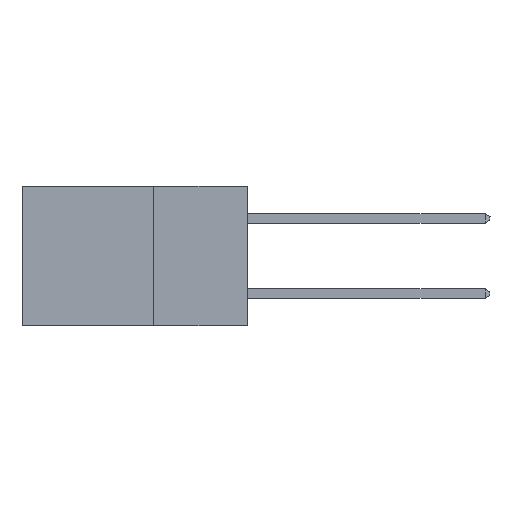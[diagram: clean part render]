
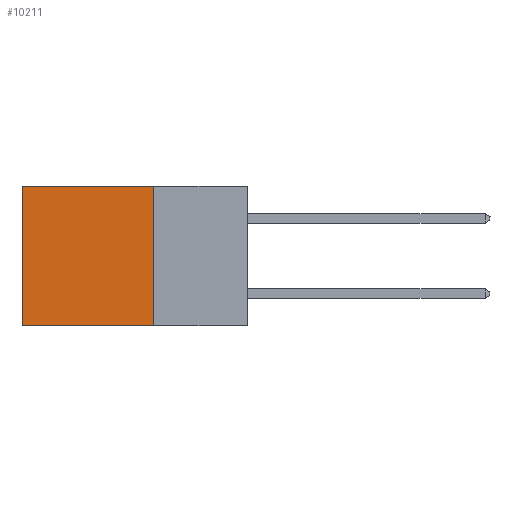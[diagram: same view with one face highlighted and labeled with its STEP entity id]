
A CAD part, left-side view. The second image highlights one B-rep face of the part: STEP entity #10211.
In plain terms, the highlighted planar face has unit normal (-1, 0, 0).
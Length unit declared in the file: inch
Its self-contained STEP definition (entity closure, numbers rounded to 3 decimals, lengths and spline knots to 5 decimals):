
#369 = CARTESIAN_POINT ( 'NONE',  ( 0.298, 0.25, 0. ) ) ;
#521 = LINE ( 'NONE', #3110, #3900 ) ;
#1960 = ORIENTED_EDGE ( 'NONE', *, *, #22011, .T. ) ;
#2977 = DIRECTION ( 'NONE',  ( 0., 0., -1. ) ) ;
#3110 = CARTESIAN_POINT ( 'NONE',  ( 0.298, 0.6, 0. ) ) ;
#3223 = EDGE_CURVE ( 'NONE', #9726, #11588, #18901, .T. ) ;
#3747 = CARTESIAN_POINT ( 'NONE',  ( 0.298, 0.25, -0.37 ) ) ;
#3900 = VECTOR ( 'NONE', #24812, 39.37008 ) ;
#4326 = ORIENTED_EDGE ( 'NONE', *, *, #6212, .F. ) ;
#4725 = EDGE_CURVE ( 'NONE', #9726, #10720, #19997, .T. ) ;
#6212 = EDGE_CURVE ( 'NONE', #10720, #7572, #20845, .T. ) ;
#7572 = VERTEX_POINT ( 'NONE', #10624 ) ;
#7655 = DIRECTION ( 'NONE',  ( 0., 1., 0. ) ) ;
#8488 = ORIENTED_EDGE ( 'NONE', *, *, #3223, .T. ) ;
#8973 = DIRECTION ( 'NONE',  ( 0., 0., -1. ) ) ;
#9197 = CARTESIAN_POINT ( 'NONE',  ( 0.298, 0.25, -0.37 ) ) ;
#9726 = VERTEX_POINT ( 'NONE', #369 ) ;
#10129 = EDGE_LOOP ( 'NONE', ( #1960, #4326, #16082, #8488 ) ) ;
#10211 = ADVANCED_FACE ( 'NONE', ( #10280 ), #20682, .F. ) ;
#10280 = FACE_OUTER_BOUND ( 'NONE', #10129, .T. ) ;
#10624 = CARTESIAN_POINT ( 'NONE',  ( 0.298, 0.6, -0.37 ) ) ;
#10720 = VERTEX_POINT ( 'NONE', #9197 ) ;
#11372 = CARTESIAN_POINT ( 'NONE',  ( 0.298, 0.25, 0. ) ) ;
#11588 = VERTEX_POINT ( 'NONE', #16580 ) ;
#12821 = DIRECTION ( 'NONE',  ( 1., 0., 0. ) ) ;
#13690 = VECTOR ( 'NONE', #15557, 39.37008 ) ;
#14196 = VECTOR ( 'NONE', #2977, 39.37008 ) ;
#15040 = VECTOR ( 'NONE', #7655, 39.37008 ) ;
#15557 = DIRECTION ( 'NONE',  ( 0., 1., 0. ) ) ;
#15786 = AXIS2_PLACEMENT_3D ( 'NONE', #16859, #12821, #8973 ) ;
#16082 = ORIENTED_EDGE ( 'NONE', *, *, #4725, .F. ) ;
#16580 = CARTESIAN_POINT ( 'NONE',  ( 0.298, 0.6, 0. ) ) ;
#16859 = CARTESIAN_POINT ( 'NONE',  ( 0.298, 0.25, 0. ) ) ;
#18901 = LINE ( 'NONE', #11372, #13690 ) ;
#19997 = LINE ( 'NONE', #22711, #14196 ) ;
#20682 = PLANE ( 'NONE',  #15786 ) ;
#20845 = LINE ( 'NONE', #3747, #15040 ) ;
#22011 = EDGE_CURVE ( 'NONE', #11588, #7572, #521, .T. ) ;
#22711 = CARTESIAN_POINT ( 'NONE',  ( 0.298, 0.25, 0. ) ) ;
#24812 = DIRECTION ( 'NONE',  ( 0., 0., -1. ) ) ;
